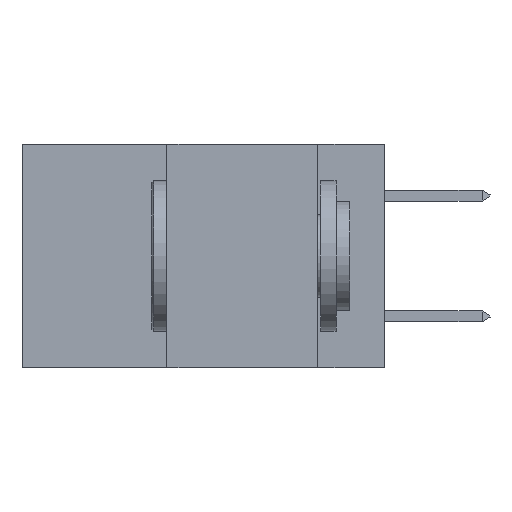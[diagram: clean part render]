
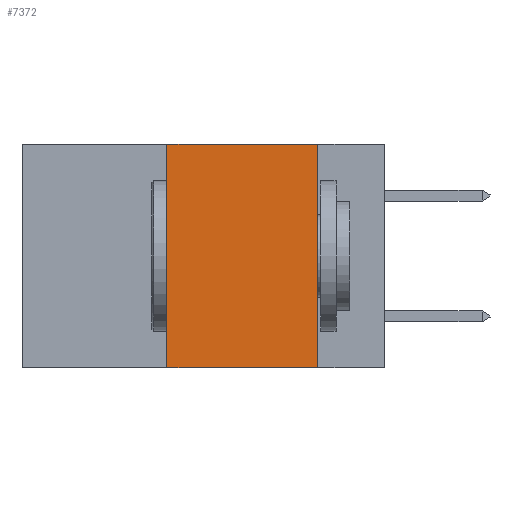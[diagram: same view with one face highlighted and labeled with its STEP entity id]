
A CAD part, left-side view. The second image highlights one B-rep face of the part: STEP entity #7372.
In plain terms, the highlighted planar face has unit normal (-1, 0, 0).
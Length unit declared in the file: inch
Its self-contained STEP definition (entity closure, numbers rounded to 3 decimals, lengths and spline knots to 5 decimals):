
#104 = VERTEX_POINT ( 'NONE', #13671 ) ;
#2594 = VECTOR ( 'NONE', #13682, 39.37008 ) ;
#5270 = EDGE_CURVE ( 'NONE', #104, #28834, #36293, .T. ) ;
#7372 = ADVANCED_FACE ( 'NONE', ( #30017 ), #26565, .F. ) ;
#9219 = LINE ( 'NONE', #26918, #28622 ) ;
#9312 = LINE ( 'NONE', #25771, #15965 ) ;
#11529 = DIRECTION ( 'NONE',  ( 0., 0., -1. ) ) ;
#11978 = DIRECTION ( 'NONE',  ( 0., -1., 0. ) ) ;
#13671 = CARTESIAN_POINT ( 'NONE',  ( 0., 0.36, -0.37 ) ) ;
#13682 = DIRECTION ( 'NONE',  ( 0., 0., 1. ) ) ;
#15829 = DIRECTION ( 'NONE',  ( 0., -1., 0. ) ) ;
#15870 = LINE ( 'NONE', #16710, #2594 ) ;
#15965 = VECTOR ( 'NONE', #37704, 39.37008 ) ;
#16375 = VERTEX_POINT ( 'NONE', #16394 ) ;
#16394 = CARTESIAN_POINT ( 'NONE',  ( 0., 0.11, 0. ) ) ;
#16710 = CARTESIAN_POINT ( 'NONE',  ( 0., 0.36, 0. ) ) ;
#17070 = ORIENTED_EDGE ( 'NONE', *, *, #5270, .T. ) ;
#17075 = ORIENTED_EDGE ( 'NONE', *, *, #24437, .F. ) ;
#17231 = DIRECTION ( 'NONE',  ( 1., 0., 0. ) ) ;
#18203 = AXIS2_PLACEMENT_3D ( 'NONE', #26609, #17231, #11529 ) ;
#19664 = VERTEX_POINT ( 'NONE', #38734 ) ;
#20146 = EDGE_LOOP ( 'NONE', ( #17075, #35000, #25464, #17070 ) ) ;
#21676 = EDGE_CURVE ( 'NONE', #19664, #16375, #9219, .T. ) ;
#24437 = EDGE_CURVE ( 'NONE', #16375, #28834, #9312, .T. ) ;
#25228 = EDGE_CURVE ( 'NONE', #104, #19664, #15870, .T. ) ;
#25464 = ORIENTED_EDGE ( 'NONE', *, *, #25228, .F. ) ;
#25771 = CARTESIAN_POINT ( 'NONE',  ( 0., 0.11, 0. ) ) ;
#26565 = PLANE ( 'NONE',  #18203 ) ;
#26609 = CARTESIAN_POINT ( 'NONE',  ( 0., 0.6, 0. ) ) ;
#26918 = CARTESIAN_POINT ( 'NONE',  ( 0., 0.6, 0. ) ) ;
#28622 = VECTOR ( 'NONE', #11978, 39.37008 ) ;
#28834 = VERTEX_POINT ( 'NONE', #31279 ) ;
#29850 = CARTESIAN_POINT ( 'NONE',  ( 0., 0.6, -0.37 ) ) ;
#30017 = FACE_OUTER_BOUND ( 'NONE', #20146, .T. ) ;
#31279 = CARTESIAN_POINT ( 'NONE',  ( 0., 0.11, -0.37 ) ) ;
#35000 = ORIENTED_EDGE ( 'NONE', *, *, #21676, .F. ) ;
#36293 = LINE ( 'NONE', #29850, #38641 ) ;
#37704 = DIRECTION ( 'NONE',  ( 0., 0., -1. ) ) ;
#38641 = VECTOR ( 'NONE', #15829, 39.37008 ) ;
#38734 = CARTESIAN_POINT ( 'NONE',  ( 0., 0.36, 0. ) ) ;
